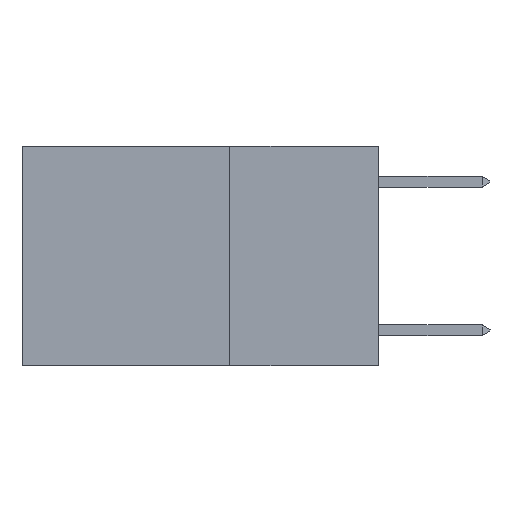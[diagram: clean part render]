
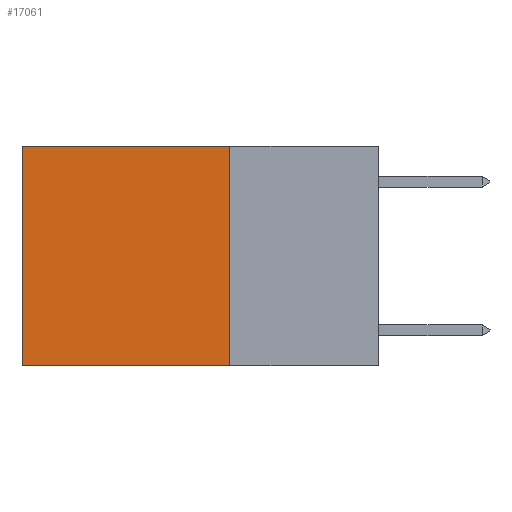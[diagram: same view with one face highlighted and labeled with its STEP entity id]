
A CAD part, left-side view. The second image highlights one B-rep face of the part: STEP entity #17061.
In plain terms, the highlighted planar face has unit normal (-1, 0, 0).
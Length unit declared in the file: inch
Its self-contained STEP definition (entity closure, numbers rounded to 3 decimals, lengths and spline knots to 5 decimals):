
#1809 = DIRECTION ( 'NONE',  ( 0., 1., 0. ) ) ;
#2029 = CARTESIAN_POINT ( 'NONE',  ( 0.2625, 0.25, 0. ) ) ;
#2637 = DIRECTION ( 'NONE',  ( 0., 1., 0. ) ) ;
#3205 = CARTESIAN_POINT ( 'NONE',  ( 0.2625, 0.25, 0. ) ) ;
#3287 = ORIENTED_EDGE ( 'NONE', *, *, #23283, .T. ) ;
#4609 = FACE_OUTER_BOUND ( 'NONE', #27835, .T. ) ;
#6400 = CARTESIAN_POINT ( 'NONE',  ( 0.2625, 0.25, 0. ) ) ;
#6961 = VERTEX_POINT ( 'NONE', #20826 ) ;
#8792 = LINE ( 'NONE', #2029, #20359 ) ;
#10286 = PLANE ( 'NONE',  #27212 ) ;
#11231 = VECTOR ( 'NONE', #2637, 39.37008 ) ;
#11336 = LINE ( 'NONE', #11930, #11231 ) ;
#11816 = VERTEX_POINT ( 'NONE', #6400 ) ;
#11930 = CARTESIAN_POINT ( 'NONE',  ( 0.2625, 0.25, -0.37 ) ) ;
#12573 = DIRECTION ( 'NONE',  ( 1., 0., 0. ) ) ;
#15908 = ORIENTED_EDGE ( 'NONE', *, *, #18040, .T. ) ;
#17061 = ADVANCED_FACE ( 'NONE', ( #4609 ), #10286, .F. ) ;
#18007 = ORIENTED_EDGE ( 'NONE', *, *, #19471, .F. ) ;
#18040 = EDGE_CURVE ( 'NONE', #18321, #22109, #22970, .T. ) ;
#18129 = EDGE_CURVE ( 'NONE', #11816, #6961, #21587, .T. ) ;
#18321 = VERTEX_POINT ( 'NONE', #19105 ) ;
#19105 = CARTESIAN_POINT ( 'NONE',  ( 0.2625, 0.6, 0. ) ) ;
#19471 = EDGE_CURVE ( 'NONE', #6961, #22109, #11336, .T. ) ;
#20359 = VECTOR ( 'NONE', #1809, 39.37008 ) ;
#20826 = CARTESIAN_POINT ( 'NONE',  ( 0.2625, 0.25, -0.37 ) ) ;
#21587 = LINE ( 'NONE', #23012, #21656 ) ;
#21656 = VECTOR ( 'NONE', #25288, 39.37008 ) ;
#22109 = VERTEX_POINT ( 'NONE', #29637 ) ;
#22173 = VECTOR ( 'NONE', #29362, 39.37008 ) ;
#22970 = LINE ( 'NONE', #29277, #22173 ) ;
#23012 = CARTESIAN_POINT ( 'NONE',  ( 0.2625, 0.25, 0. ) ) ;
#23283 = EDGE_CURVE ( 'NONE', #11816, #18321, #8792, .T. ) ;
#23414 = ORIENTED_EDGE ( 'NONE', *, *, #18129, .F. ) ;
#25288 = DIRECTION ( 'NONE',  ( 0., 0., -1. ) ) ;
#27212 = AXIS2_PLACEMENT_3D ( 'NONE', #3205, #12573, #28469 ) ;
#27835 = EDGE_LOOP ( 'NONE', ( #15908, #18007, #23414, #3287 ) ) ;
#28469 = DIRECTION ( 'NONE',  ( 0., 0., -1. ) ) ;
#29277 = CARTESIAN_POINT ( 'NONE',  ( 0.2625, 0.6, 0. ) ) ;
#29362 = DIRECTION ( 'NONE',  ( 0., 0., -1. ) ) ;
#29637 = CARTESIAN_POINT ( 'NONE',  ( 0.2625, 0.6, -0.37 ) ) ;
